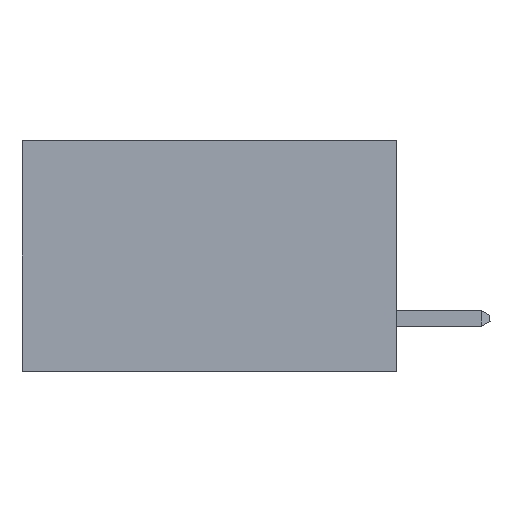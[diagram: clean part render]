
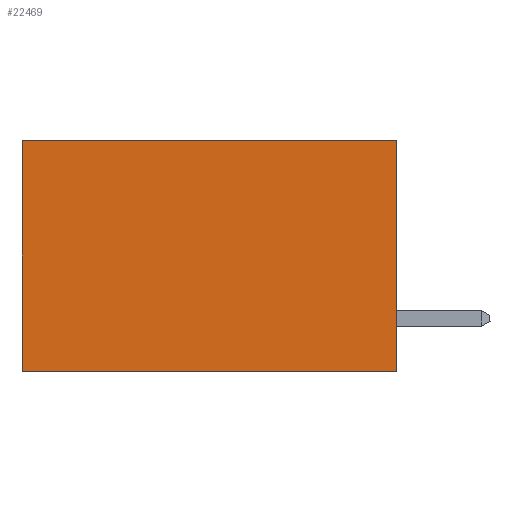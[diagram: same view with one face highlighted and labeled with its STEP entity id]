
A CAD part, left-side view. The second image highlights one B-rep face of the part: STEP entity #22469.
In plain terms, the highlighted planar face has unit normal (-1, 0, 0).
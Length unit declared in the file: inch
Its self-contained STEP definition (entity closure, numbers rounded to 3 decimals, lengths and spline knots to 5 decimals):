
#540 = LINE ( 'NONE', #16241, #14749 ) ;
#2998 = EDGE_CURVE ( 'NONE', #20914, #14109, #8052, .T. ) ;
#3097 = EDGE_CURVE ( 'NONE', #20914, #19859, #7219, .T. ) ;
#3153 = DIRECTION ( 'NONE',  ( 0., 1., 0. ) ) ;
#3233 = CARTESIAN_POINT ( 'NONE',  ( 0.298, 0.6, 0. ) ) ;
#4011 = ORIENTED_EDGE ( 'NONE', *, *, #2998, .T. ) ;
#4441 = VECTOR ( 'NONE', #3153, 39.37008 ) ;
#4651 = LINE ( 'NONE', #7043, #6039 ) ;
#5464 = CARTESIAN_POINT ( 'NONE',  ( 0.298, 0., 0. ) ) ;
#6039 = VECTOR ( 'NONE', #8809, 39.37008 ) ;
#6543 = PLANE ( 'NONE',  #18729 ) ;
#7043 = CARTESIAN_POINT ( 'NONE',  ( 0.298, 0.6, 0. ) ) ;
#7219 = LINE ( 'NONE', #5464, #21626 ) ;
#7221 = CARTESIAN_POINT ( 'NONE',  ( 0.298, 0., 0. ) ) ;
#7888 = CARTESIAN_POINT ( 'NONE',  ( 0.298, 0., -0.37 ) ) ;
#8052 = LINE ( 'NONE', #13884, #4441 ) ;
#8291 = ORIENTED_EDGE ( 'NONE', *, *, #14629, .F. ) ;
#8453 = ORIENTED_EDGE ( 'NONE', *, *, #19567, .T. ) ;
#8483 = DIRECTION ( 'NONE',  ( 1., 0., 0. ) ) ;
#8809 = DIRECTION ( 'NONE',  ( 0., 0., -1. ) ) ;
#10734 = EDGE_LOOP ( 'NONE', ( #8453, #8291, #22711, #4011 ) ) ;
#11951 = DIRECTION ( 'NONE',  ( 0., 1., 0. ) ) ;
#13884 = CARTESIAN_POINT ( 'NONE',  ( 0.298, 0., 0. ) ) ;
#14109 = VERTEX_POINT ( 'NONE', #3233 ) ;
#14629 = EDGE_CURVE ( 'NONE', #19859, #15842, #540, .T. ) ;
#14749 = VECTOR ( 'NONE', #11951, 39.37008 ) ;
#15402 = CARTESIAN_POINT ( 'NONE',  ( 0.298, 0.6, -0.37 ) ) ;
#15842 = VERTEX_POINT ( 'NONE', #15402 ) ;
#16241 = CARTESIAN_POINT ( 'NONE',  ( 0.298, 0., -0.37 ) ) ;
#17358 = CARTESIAN_POINT ( 'NONE',  ( 0.298, 0., 0. ) ) ;
#18729 = AXIS2_PLACEMENT_3D ( 'NONE', #17358, #8483, #22710 ) ;
#19567 = EDGE_CURVE ( 'NONE', #14109, #15842, #4651, .T. ) ;
#19859 = VERTEX_POINT ( 'NONE', #7888 ) ;
#20334 = FACE_OUTER_BOUND ( 'NONE', #10734, .T. ) ;
#20914 = VERTEX_POINT ( 'NONE', #7221 ) ;
#21626 = VECTOR ( 'NONE', #22969, 39.37008 ) ;
#22469 = ADVANCED_FACE ( 'NONE', ( #20334 ), #6543, .F. ) ;
#22710 = DIRECTION ( 'NONE',  ( 0., 0., -1. ) ) ;
#22711 = ORIENTED_EDGE ( 'NONE', *, *, #3097, .F. ) ;
#22969 = DIRECTION ( 'NONE',  ( 0., 0., -1. ) ) ;
